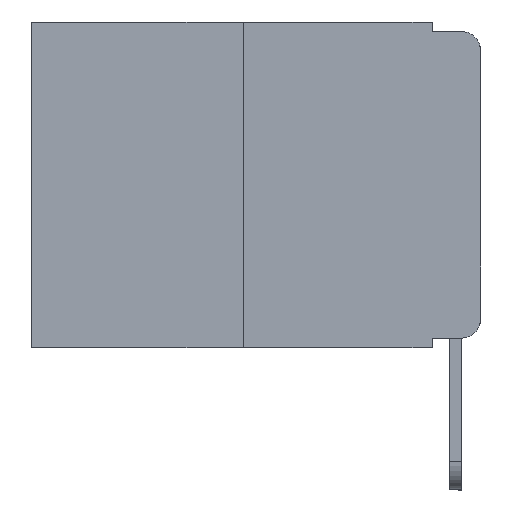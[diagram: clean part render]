
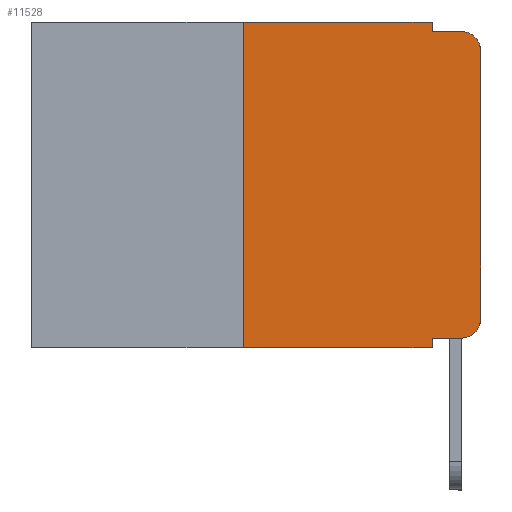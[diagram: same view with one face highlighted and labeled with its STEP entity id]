
A CAD part, left-side view. The second image highlights one B-rep face of the part: STEP entity #11528.
In plain terms, the highlighted planar face has unit normal (-1, 0, 0).
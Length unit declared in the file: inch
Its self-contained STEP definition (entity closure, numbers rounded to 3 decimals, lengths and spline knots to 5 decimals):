
#5 = CARTESIAN_POINT ( 'NONE',  ( 0., 0.051, -0.01 ) ) ;
#379 = DIRECTION ( 'NONE',  ( 0., 0., -1. ) ) ;
#942 = EDGE_CURVE ( 'NONE', #11712, #4607, #17199, .T. ) ;
#967 = VECTOR ( 'NONE', #12165, 39.37008 ) ;
#1250 = CARTESIAN_POINT ( 'NONE',  ( 0., 0.051, 0. ) ) ;
#1803 = ORIENTED_EDGE ( 'NONE', *, *, #15865, .T. ) ;
#1877 = ORIENTED_EDGE ( 'NONE', *, *, #16964, .F. ) ;
#1933 = CARTESIAN_POINT ( 'NONE',  ( 0., 0.02, -0.333 ) ) ;
#2105 = DIRECTION ( 'NONE',  ( 0., -1., 0. ) ) ;
#2133 = VECTOR ( 'NONE', #2105, 39.37008 ) ;
#2840 = VERTEX_POINT ( 'NONE', #6322 ) ;
#3006 = EDGE_CURVE ( 'NONE', #10565, #5311, #19431, .T. ) ;
#3185 = LINE ( 'NONE', #4701, #9300 ) ;
#3192 = VECTOR ( 'NONE', #19225, 39.37008 ) ;
#3250 = CARTESIAN_POINT ( 'NONE',  ( 0., 0.051, -0.333 ) ) ;
#3826 = DIRECTION ( 'NONE',  ( 0., 0., -1. ) ) ;
#4266 = CARTESIAN_POINT ( 'NONE',  ( 0., 0.051, 0. ) ) ;
#4282 = DIRECTION ( 'NONE',  ( 0., 0., -1. ) ) ;
#4607 = VERTEX_POINT ( 'NONE', #6836 ) ;
#4701 = CARTESIAN_POINT ( 'NONE',  ( 0., 0.473, 0. ) ) ;
#4935 = ORIENTED_EDGE ( 'NONE', *, *, #20547, .F. ) ;
#5168 = DIRECTION ( 'NONE',  ( 0., -1., 0. ) ) ;
#5311 = VERTEX_POINT ( 'NONE', #13103 ) ;
#5645 = ORIENTED_EDGE ( 'NONE', *, *, #7141, .F. ) ;
#6311 = CARTESIAN_POINT ( 'NONE',  ( 0., 0.25, 0. ) ) ;
#6322 = CARTESIAN_POINT ( 'NONE',  ( 0., 0.25, -0.343 ) ) ;
#6399 = VECTOR ( 'NONE', #379, 39.37008 ) ;
#6659 = CIRCLE ( 'NONE', #17448, 0.02 ) ;
#6740 = EDGE_CURVE ( 'NONE', #2840, #20904, #20995, .T. ) ;
#6767 = LINE ( 'NONE', #8395, #3192 ) ;
#6836 = CARTESIAN_POINT ( 'NONE',  ( 0., 0.051, -0.01 ) ) ;
#7141 = EDGE_CURVE ( 'NONE', #4607, #10858, #17698, .T. ) ;
#7270 = CARTESIAN_POINT ( 'NONE',  ( 0., 0.051, 0. ) ) ;
#7414 = AXIS2_PLACEMENT_3D ( 'NONE', #14180, #14067, #3826 ) ;
#8395 = CARTESIAN_POINT ( 'NONE',  ( 0., 0.25, 0. ) ) ;
#8476 = FACE_OUTER_BOUND ( 'NONE', #17542, .T. ) ;
#8798 = EDGE_CURVE ( 'NONE', #5311, #10858, #6659, .T. ) ;
#9142 = LINE ( 'NONE', #7270, #12198 ) ;
#9300 = VECTOR ( 'NONE', #10285, 39.37008 ) ;
#9418 = EDGE_CURVE ( 'NONE', #21142, #11712, #3185, .T. ) ;
#9749 = AXIS2_PLACEMENT_3D ( 'NONE', #14612, #21278, #12199 ) ;
#10285 = DIRECTION ( 'NONE',  ( 0., -1., 0. ) ) ;
#10469 = ORIENTED_EDGE ( 'NONE', *, *, #6740, .T. ) ;
#10565 = VERTEX_POINT ( 'NONE', #13444 ) ;
#10649 = LINE ( 'NONE', #12398, #967 ) ;
#10858 = VERTEX_POINT ( 'NONE', #20067 ) ;
#11499 = VERTEX_POINT ( 'NONE', #3250 ) ;
#11528 = ADVANCED_FACE ( 'NONE', ( #8476 ), #22691, .F. ) ;
#11712 = VERTEX_POINT ( 'NONE', #4266 ) ;
#11920 = CARTESIAN_POINT ( 'NONE',  ( 0., 0.051, -0.343 ) ) ;
#12165 = DIRECTION ( 'NONE',  ( 0., -1., 0. ) ) ;
#12198 = VECTOR ( 'NONE', #19853, 39.37008 ) ;
#12199 = DIRECTION ( 'NONE',  ( 0., 0., -1. ) ) ;
#12398 = CARTESIAN_POINT ( 'NONE',  ( 0., 0.051, -0.333 ) ) ;
#12793 = DIRECTION ( 'NONE',  ( 0., 0., 1. ) ) ;
#13103 = CARTESIAN_POINT ( 'NONE',  ( 0., 0., -0.03 ) ) ;
#13238 = CARTESIAN_POINT ( 'NONE',  ( 0., 0.02, -0.03 ) ) ;
#13444 = CARTESIAN_POINT ( 'NONE',  ( 0., 0., -0.313 ) ) ;
#14067 = DIRECTION ( 'NONE',  ( -1., 0., 0. ) ) ;
#14180 = CARTESIAN_POINT ( 'NONE',  ( 0., 0.02, -0.313 ) ) ;
#14612 = CARTESIAN_POINT ( 'NONE',  ( 0., 0.473, 0. ) ) ;
#15865 = EDGE_CURVE ( 'NONE', #11499, #20559, #10649, .T. ) ;
#15937 = ORIENTED_EDGE ( 'NONE', *, *, #9418, .F. ) ;
#16149 = ORIENTED_EDGE ( 'NONE', *, *, #3006, .T. ) ;
#16616 = DIRECTION ( 'NONE',  ( -1., 0., 0. ) ) ;
#16964 = EDGE_CURVE ( 'NONE', #2840, #21142, #6767, .T. ) ;
#17199 = LINE ( 'NONE', #1250, #6399 ) ;
#17448 = AXIS2_PLACEMENT_3D ( 'NONE', #13238, #16616, #4282 ) ;
#17542 = EDGE_LOOP ( 'NONE', ( #16149, #22313, #5645, #19900, #15937, #1877, #10469, #4935, #1803, #21801 ) ) ;
#17698 = LINE ( 'NONE', #5, #2133 ) ;
#18933 = CIRCLE ( 'NONE', #7414, 0.02 ) ;
#19225 = DIRECTION ( 'NONE',  ( 0., 0., 1. ) ) ;
#19431 = LINE ( 'NONE', #21524, #22408 ) ;
#19853 = DIRECTION ( 'NONE',  ( 0., 0., -1. ) ) ;
#19900 = ORIENTED_EDGE ( 'NONE', *, *, #942, .F. ) ;
#20067 = CARTESIAN_POINT ( 'NONE',  ( 0., 0.02, -0.01 ) ) ;
#20547 = EDGE_CURVE ( 'NONE', #11499, #20904, #9142, .T. ) ;
#20559 = VERTEX_POINT ( 'NONE', #1933 ) ;
#20702 = VECTOR ( 'NONE', #5168, 39.37008 ) ;
#20904 = VERTEX_POINT ( 'NONE', #11920 ) ;
#20995 = LINE ( 'NONE', #21109, #20702 ) ;
#21109 = CARTESIAN_POINT ( 'NONE',  ( 0., 0.473, -0.343 ) ) ;
#21142 = VERTEX_POINT ( 'NONE', #6311 ) ;
#21278 = DIRECTION ( 'NONE',  ( 1., 0., 0. ) ) ;
#21524 = CARTESIAN_POINT ( 'NONE',  ( 0., 0., 0. ) ) ;
#21801 = ORIENTED_EDGE ( 'NONE', *, *, #21855, .T. ) ;
#21855 = EDGE_CURVE ( 'NONE', #20559, #10565, #18933, .T. ) ;
#22313 = ORIENTED_EDGE ( 'NONE', *, *, #8798, .T. ) ;
#22408 = VECTOR ( 'NONE', #12793, 39.37008 ) ;
#22691 = PLANE ( 'NONE',  #9749 ) ;
